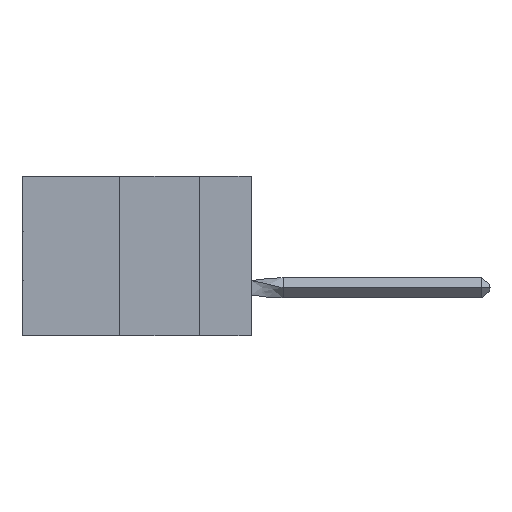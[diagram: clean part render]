
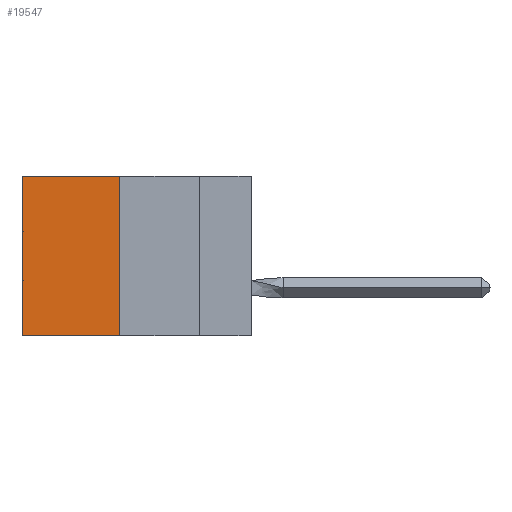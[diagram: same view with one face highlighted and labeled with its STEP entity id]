
A CAD part, left-side view. The second image highlights one B-rep face of the part: STEP entity #19547.
In plain terms, the highlighted planar face has unit normal (-1, 0, 0).
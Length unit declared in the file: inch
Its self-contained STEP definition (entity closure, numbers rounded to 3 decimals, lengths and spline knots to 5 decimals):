
#481 = CARTESIAN_POINT ( 'NONE',  ( 0.305, 0.72, -0.5 ) ) ;
#2826 = VECTOR ( 'NONE', #26464, 39.37008 ) ;
#3186 = VERTEX_POINT ( 'NONE', #20547 ) ;
#6439 = VERTEX_POINT ( 'NONE', #42765 ) ;
#7206 = CARTESIAN_POINT ( 'NONE',  ( 0.305, 0.413, 0. ) ) ;
#12337 = VECTOR ( 'NONE', #14407, 39.37008 ) ;
#13293 = EDGE_CURVE ( 'NONE', #3186, #6439, #19033, .T. ) ;
#14407 = DIRECTION ( 'NONE',  ( 0., 0., -1. ) ) ;
#14961 = VECTOR ( 'NONE', #40561, 39.37008 ) ;
#15368 = EDGE_CURVE ( 'NONE', #30469, #26488, #44662, .T. ) ;
#15828 = LINE ( 'NONE', #21741, #12337 ) ;
#17724 = DIRECTION ( 'NONE',  ( 0., 0., -1. ) ) ;
#19033 = LINE ( 'NONE', #7206, #2826 ) ;
#19547 = ADVANCED_FACE ( 'NONE', ( #25065 ), #47242, .F. ) ;
#20547 = CARTESIAN_POINT ( 'NONE',  ( 0.305, 0.413, 0. ) ) ;
#21741 = CARTESIAN_POINT ( 'NONE',  ( 0.305, 0.413, -0.5 ) ) ;
#24019 = ORIENTED_EDGE ( 'NONE', *, *, #15368, .F. ) ;
#24262 = CARTESIAN_POINT ( 'NONE',  ( 0.305, 0.72, -0.5 ) ) ;
#24492 = DIRECTION ( 'NONE',  ( 1., 0., 0. ) ) ;
#24956 = CARTESIAN_POINT ( 'NONE',  ( 0.305, 0.413, -0.5 ) ) ;
#25065 = FACE_OUTER_BOUND ( 'NONE', #25795, .T. ) ;
#25742 = CARTESIAN_POINT ( 'NONE',  ( 0.305, 0.413, -0.5 ) ) ;
#25795 = EDGE_LOOP ( 'NONE', ( #26172, #24019, #45437, #37392 ) ) ;
#26172 = ORIENTED_EDGE ( 'NONE', *, *, #39830, .T. ) ;
#26464 = DIRECTION ( 'NONE',  ( 0., 1., 0. ) ) ;
#26488 = VERTEX_POINT ( 'NONE', #481 ) ;
#30469 = VERTEX_POINT ( 'NONE', #41637 ) ;
#35683 = AXIS2_PLACEMENT_3D ( 'NONE', #24956, #24492, #36010 ) ;
#36010 = DIRECTION ( 'NONE',  ( 0., 0., -1. ) ) ;
#36487 = VECTOR ( 'NONE', #17724, 39.37008 ) ;
#37392 = ORIENTED_EDGE ( 'NONE', *, *, #13293, .T. ) ;
#39830 = EDGE_CURVE ( 'NONE', #6439, #26488, #46411, .T. ) ;
#40561 = DIRECTION ( 'NONE',  ( 0., 1., 0. ) ) ;
#41637 = CARTESIAN_POINT ( 'NONE',  ( 0.305, 0.413, -0.5 ) ) ;
#42765 = CARTESIAN_POINT ( 'NONE',  ( 0.305, 0.72, 0. ) ) ;
#43643 = EDGE_CURVE ( 'NONE', #3186, #30469, #15828, .T. ) ;
#44662 = LINE ( 'NONE', #25742, #14961 ) ;
#45437 = ORIENTED_EDGE ( 'NONE', *, *, #43643, .F. ) ;
#46411 = LINE ( 'NONE', #24262, #36487 ) ;
#47242 = PLANE ( 'NONE',  #35683 ) ;
